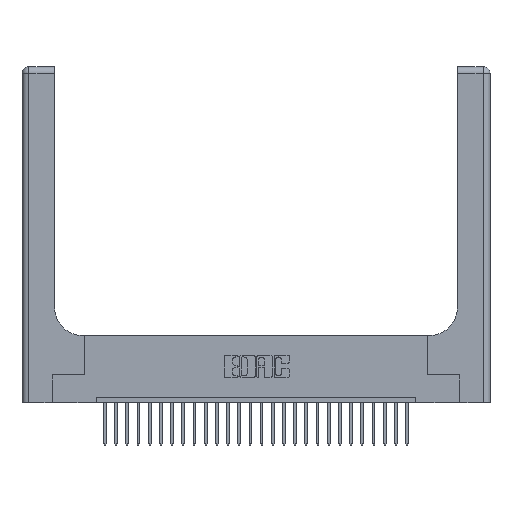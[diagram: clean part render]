
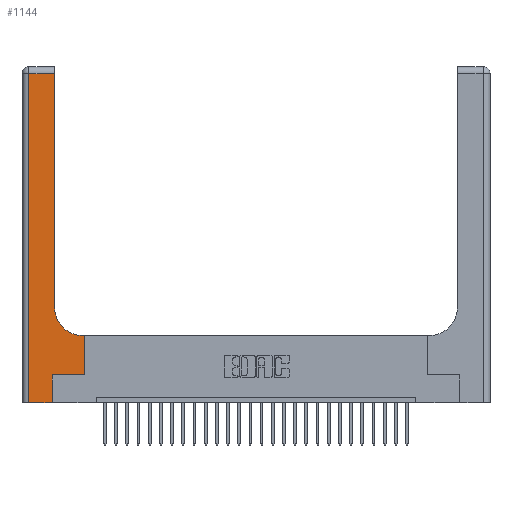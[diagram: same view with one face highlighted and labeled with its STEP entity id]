
A CAD part, top view. The second image highlights one B-rep face of the part: STEP entity #1144.
In plain terms, the highlighted planar face has unit normal (0, 0, 1).
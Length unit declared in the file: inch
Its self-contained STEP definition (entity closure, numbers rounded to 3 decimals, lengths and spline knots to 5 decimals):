
#72 = DIRECTION ( 'NONE',  ( -1., 0., 0. ) ) ;
#606 = CARTESIAN_POINT ( 'NONE',  ( 0.5585, 0.25, 0.37 ) ) ;
#829 = VECTOR ( 'NONE', #9608, 39.37008 ) ;
#1144 = ADVANCED_FACE ( 'NONE', ( #19892 ), #21170, .F. ) ;
#1907 = EDGE_CURVE ( 'NONE', #10841, #22123, #10044, .T. ) ;
#2548 = CARTESIAN_POINT ( 'NONE',  ( 0.5585, 0.6, 0.37 ) ) ;
#2728 = ORIENTED_EDGE ( 'NONE', *, *, #8174, .T. ) ;
#2860 = VECTOR ( 'NONE', #14846, 39.37008 ) ;
#3680 = VECTOR ( 'NONE', #19199, 39.37008 ) ;
#4164 = CARTESIAN_POINT ( 'NONE',  ( 0.269, 0., 0.37 ) ) ;
#5008 = VERTEX_POINT ( 'NONE', #606 ) ;
#5213 = VECTOR ( 'NONE', #9548, 39.37008 ) ;
#5484 = VECTOR ( 'NONE', #16173, 39.37008 ) ;
#5622 = VERTEX_POINT ( 'NONE', #2548 ) ;
#6377 = EDGE_CURVE ( 'NONE', #5008, #5622, #25206, .T. ) ;
#6435 = VERTEX_POINT ( 'NONE', #25921 ) ;
#6673 = EDGE_CURVE ( 'NONE', #7023, #27691, #12653, .T. ) ;
#6777 = LINE ( 'NONE', #17409, #3680 ) ;
#6882 = EDGE_LOOP ( 'NONE', ( #17591, #2728, #27562, #13627, #19601, #20713, #7883, #15767, #15354 ) ) ;
#7023 = VERTEX_POINT ( 'NONE', #7845 ) ;
#7345 = LINE ( 'NONE', #20557, #829 ) ;
#7453 = LINE ( 'NONE', #25881, #27107 ) ;
#7583 = CARTESIAN_POINT ( 'NONE',  ( 0.5415, 0.6, 0.37 ) ) ;
#7845 = CARTESIAN_POINT ( 'NONE',  ( 0.2915, 0.85, 0.37 ) ) ;
#7883 = ORIENTED_EDGE ( 'NONE', *, *, #6377, .T. ) ;
#8174 = EDGE_CURVE ( 'NONE', #27691, #6435, #7453, .T. ) ;
#8672 = CARTESIAN_POINT ( 'NONE',  ( 0.5585, 0.25, 0.37 ) ) ;
#9548 = DIRECTION ( 'NONE',  ( 1., 0., 0. ) ) ;
#9608 = DIRECTION ( 'NONE',  ( 1., 0., 0. ) ) ;
#9644 = CARTESIAN_POINT ( 'NONE',  ( 0.2915, 3., 0.37 ) ) ;
#9931 = DIRECTION ( 'NONE',  ( 0., 0., -1. ) ) ;
#10028 = VERTEX_POINT ( 'NONE', #25042 ) ;
#10044 = LINE ( 'NONE', #19402, #2860 ) ;
#10841 = VERTEX_POINT ( 'NONE', #4164 ) ;
#11027 = LINE ( 'NONE', #11648, #5213 ) ;
#11029 = CARTESIAN_POINT ( 'NONE',  ( 0.2915, 2.94, 0.37 ) ) ;
#11389 = CARTESIAN_POINT ( 'NONE',  ( 0.5415, 0.85, 0.37 ) ) ;
#11648 = CARTESIAN_POINT ( 'NONE',  ( 0., 0., 0.37 ) ) ;
#12653 = LINE ( 'NONE', #9644, #5484 ) ;
#13532 = DIRECTION ( 'NONE',  ( 0., 0., -1. ) ) ;
#13627 = ORIENTED_EDGE ( 'NONE', *, *, #23775, .T. ) ;
#13640 = DIRECTION ( 'NONE',  ( 0., 1., 0. ) ) ;
#14262 = DIRECTION ( 'NONE',  ( -1., 0., 0. ) ) ;
#14846 = DIRECTION ( 'NONE',  ( 0., 1., 0. ) ) ;
#15354 = ORIENTED_EDGE ( 'NONE', *, *, #26726, .T. ) ;
#15767 = ORIENTED_EDGE ( 'NONE', *, *, #21174, .T. ) ;
#15971 = EDGE_CURVE ( 'NONE', #22123, #5008, #7345, .T. ) ;
#16173 = DIRECTION ( 'NONE',  ( 0., 1., 0. ) ) ;
#16465 = CARTESIAN_POINT ( 'NONE',  ( 0., 3., 0.37 ) ) ;
#17312 = CARTESIAN_POINT ( 'NONE',  ( 0.2915, 0.6, 0.37 ) ) ;
#17409 = CARTESIAN_POINT ( 'NONE',  ( 0.06, 3., 0.37 ) ) ;
#17591 = ORIENTED_EDGE ( 'NONE', *, *, #6673, .T. ) ;
#19199 = DIRECTION ( 'NONE',  ( 0., -1., 0. ) ) ;
#19402 = CARTESIAN_POINT ( 'NONE',  ( 0.269, 0., 0.37 ) ) ;
#19425 = VECTOR ( 'NONE', #13640, 39.37008 ) ;
#19601 = ORIENTED_EDGE ( 'NONE', *, *, #1907, .T. ) ;
#19892 = FACE_OUTER_BOUND ( 'NONE', #6882, .T. ) ;
#20557 = CARTESIAN_POINT ( 'NONE',  ( 0.269, 0.25, 0.37 ) ) ;
#20713 = ORIENTED_EDGE ( 'NONE', *, *, #15971, .T. ) ;
#21170 = PLANE ( 'NONE',  #27247 ) ;
#21174 = EDGE_CURVE ( 'NONE', #5622, #28056, #24700, .T. ) ;
#22123 = VERTEX_POINT ( 'NONE', #23739 ) ;
#22636 = VECTOR ( 'NONE', #72, 39.37008 ) ;
#23739 = CARTESIAN_POINT ( 'NONE',  ( 0.269, 0.25, 0.37 ) ) ;
#23775 = EDGE_CURVE ( 'NONE', #10028, #10841, #11027, .T. ) ;
#24700 = LINE ( 'NONE', #17312, #22636 ) ;
#25042 = CARTESIAN_POINT ( 'NONE',  ( 0.06, 0., 0.37 ) ) ;
#25206 = LINE ( 'NONE', #8672, #19425 ) ;
#25881 = CARTESIAN_POINT ( 'NONE',  ( 0., 2.94, 0.37 ) ) ;
#25921 = CARTESIAN_POINT ( 'NONE',  ( 0.06, 2.94, 0.37 ) ) ;
#25971 = DIRECTION ( 'NONE',  ( -1., 0., 0. ) ) ;
#26132 = CIRCLE ( 'NONE', #27975, 0.25 ) ;
#26698 = DIRECTION ( 'NONE',  ( 1., 0., 0. ) ) ;
#26726 = EDGE_CURVE ( 'NONE', #28056, #7023, #26132, .T. ) ;
#27107 = VECTOR ( 'NONE', #25971, 39.37008 ) ;
#27145 = EDGE_CURVE ( 'NONE', #6435, #10028, #6777, .T. ) ;
#27247 = AXIS2_PLACEMENT_3D ( 'NONE', #16465, #9931, #14262 ) ;
#27562 = ORIENTED_EDGE ( 'NONE', *, *, #27145, .T. ) ;
#27691 = VERTEX_POINT ( 'NONE', #11029 ) ;
#27975 = AXIS2_PLACEMENT_3D ( 'NONE', #11389, #13532, #26698 ) ;
#28056 = VERTEX_POINT ( 'NONE', #7583 ) ;
